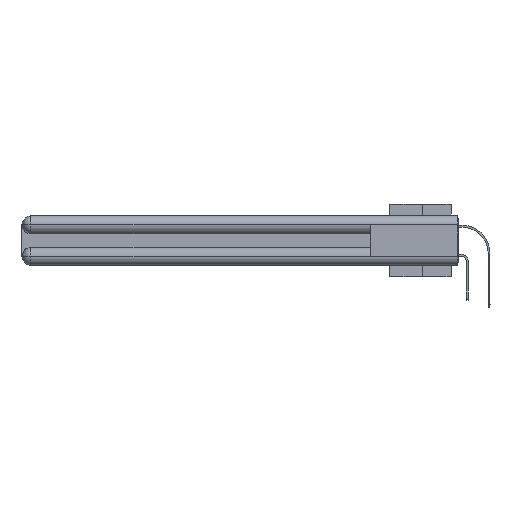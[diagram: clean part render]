
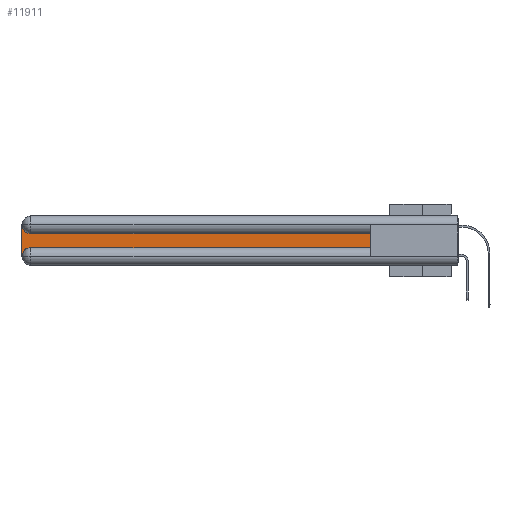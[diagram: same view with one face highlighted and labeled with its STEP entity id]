
A CAD part, left-side view. The second image highlights one B-rep face of the part: STEP entity #11911.
In plain terms, the highlighted planar face has unit normal (-1, 0, 0).
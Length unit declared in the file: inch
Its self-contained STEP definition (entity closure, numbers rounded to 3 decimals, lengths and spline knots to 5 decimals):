
#315 = FACE_OUTER_BOUND ( 'NONE', #32338, .T. ) ;
#335 = DIRECTION ( 'NONE',  ( 1., 0., 0. ) ) ;
#775 = VERTEX_POINT ( 'NONE', #2131 ) ;
#872 = DIRECTION ( 'NONE',  ( 1., 0., 0. ) ) ;
#1385 = CARTESIAN_POINT ( 'NONE',  ( 0.075, 0.6, -0.2175 ) ) ;
#1628 = VERTEX_POINT ( 'NONE', #24638 ) ;
#2131 = CARTESIAN_POINT ( 'NONE',  ( 0.075, 0.6, -0.1225 ) ) ;
#2316 = ORIENTED_EDGE ( 'NONE', *, *, #27388, .T. ) ;
#3249 = ORIENTED_EDGE ( 'NONE', *, *, #11189, .T. ) ;
#3642 = LINE ( 'NONE', #1385, #31617 ) ;
#5567 = VERTEX_POINT ( 'NONE', #22213 ) ;
#6781 = EDGE_CURVE ( 'NONE', #775, #5567, #27125, .T. ) ;
#6978 = VECTOR ( 'NONE', #11027, 39.37008 ) ;
#7434 = AXIS2_PLACEMENT_3D ( 'NONE', #33377, #33919, #34106 ) ;
#8047 = CIRCLE ( 'NONE', #7434, 0.06 ) ;
#8169 = ORIENTED_EDGE ( 'NONE', *, *, #29523, .T. ) ;
#9913 = VERTEX_POINT ( 'NONE', #22026 ) ;
#11027 = DIRECTION ( 'NONE',  ( 0., 0., -1. ) ) ;
#11189 = EDGE_CURVE ( 'NONE', #19431, #9913, #3642, .T. ) ;
#11666 = LINE ( 'NONE', #23039, #19478 ) ;
#11911 = ADVANCED_FACE ( 'NONE', ( #315 ), #17657, .F. ) ;
#15063 = DIRECTION ( 'NONE',  ( 0., 0., -1. ) ) ;
#17657 = PLANE ( 'NONE',  #23301 ) ;
#17732 = EDGE_CURVE ( 'NONE', #9913, #775, #11666, .T. ) ;
#18547 = DIRECTION ( 'NONE',  ( 0., 1., 0. ) ) ;
#19431 = VERTEX_POINT ( 'NONE', #23198 ) ;
#19478 = VECTOR ( 'NONE', #34438, 39.37008 ) ;
#22026 = CARTESIAN_POINT ( 'NONE',  ( 0.075, 0.6, -0.2175 ) ) ;
#22066 = VERTEX_POINT ( 'NONE', #35512 ) ;
#22213 = CARTESIAN_POINT ( 'NONE',  ( 0.075, 2.94, -0.1225 ) ) ;
#23039 = CARTESIAN_POINT ( 'NONE',  ( 0.075, 0.6, -0.2175 ) ) ;
#23198 = CARTESIAN_POINT ( 'NONE',  ( 0.075, 2.94, -0.2175 ) ) ;
#23301 = AXIS2_PLACEMENT_3D ( 'NONE', #26438, #872, #23627 ) ;
#23627 = DIRECTION ( 'NONE',  ( 0., 0., -1. ) ) ;
#24638 = CARTESIAN_POINT ( 'NONE',  ( 0.075, 3., -0.0625 ) ) ;
#24829 = ORIENTED_EDGE ( 'NONE', *, *, #35453, .T. ) ;
#24929 = VECTOR ( 'NONE', #18547, 39.37008 ) ;
#24979 = CIRCLE ( 'NONE', #35088, 0.06 ) ;
#26438 = CARTESIAN_POINT ( 'NONE',  ( 0.075, 3., -0.1225 ) ) ;
#27125 = LINE ( 'NONE', #33100, #24929 ) ;
#27336 = ORIENTED_EDGE ( 'NONE', *, *, #6781, .T. ) ;
#27388 = EDGE_CURVE ( 'NONE', #22066, #19431, #24979, .T. ) ;
#28021 = CARTESIAN_POINT ( 'NONE',  ( 0.075, 3., -0.2175 ) ) ;
#29523 = EDGE_CURVE ( 'NONE', #5567, #1628, #8047, .T. ) ;
#31617 = VECTOR ( 'NONE', #32355, 39.37008 ) ;
#32338 = EDGE_LOOP ( 'NONE', ( #27336, #8169, #24829, #2316, #3249, #33927 ) ) ;
#32355 = DIRECTION ( 'NONE',  ( 0., -1., 0. ) ) ;
#33100 = CARTESIAN_POINT ( 'NONE',  ( 0.075, 0.6, -0.1225 ) ) ;
#33377 = CARTESIAN_POINT ( 'NONE',  ( 0.075, 2.94, -0.0625 ) ) ;
#33447 = LINE ( 'NONE', #28021, #6978 ) ;
#33919 = DIRECTION ( 'NONE',  ( 1., 0., 0. ) ) ;
#33927 = ORIENTED_EDGE ( 'NONE', *, *, #17732, .T. ) ;
#34106 = DIRECTION ( 'NONE',  ( 0., 0., -1. ) ) ;
#34438 = DIRECTION ( 'NONE',  ( 0., 0., 1. ) ) ;
#35088 = AXIS2_PLACEMENT_3D ( 'NONE', #35228, #335, #15063 ) ;
#35228 = CARTESIAN_POINT ( 'NONE',  ( 0.075, 2.94, -0.2775 ) ) ;
#35453 = EDGE_CURVE ( 'NONE', #1628, #22066, #33447, .T. ) ;
#35512 = CARTESIAN_POINT ( 'NONE',  ( 0.075, 3., -0.2775 ) ) ;
